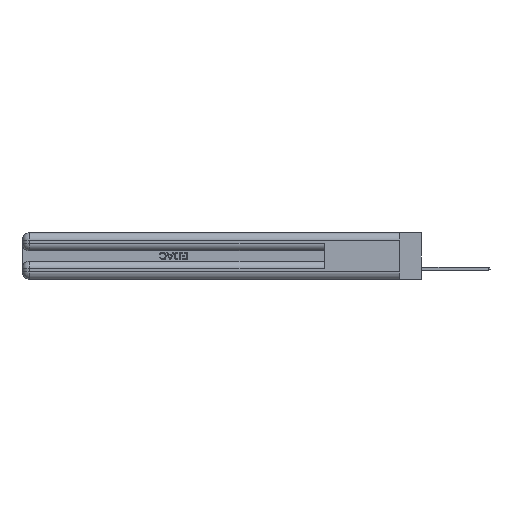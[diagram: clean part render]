
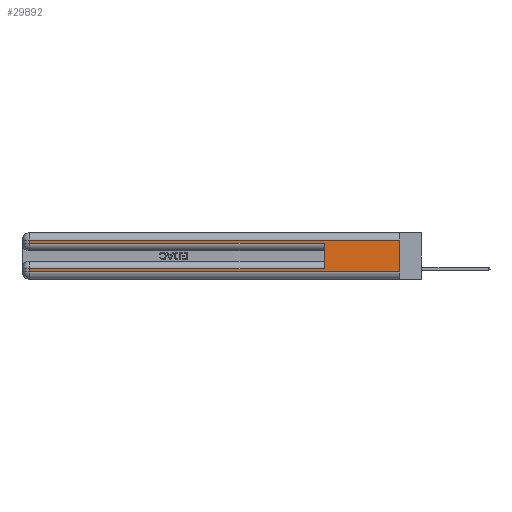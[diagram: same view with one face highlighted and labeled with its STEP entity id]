
A CAD part, left-side view. The second image highlights one B-rep face of the part: STEP entity #29892.
In plain terms, the highlighted planar face has unit normal (-1, 0, 0).
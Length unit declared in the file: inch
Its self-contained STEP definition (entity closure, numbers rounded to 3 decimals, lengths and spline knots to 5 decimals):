
#264 = ORIENTED_EDGE ( 'NONE', *, *, #24487, .T. ) ;
#541 = VECTOR ( 'NONE', #41531, 39.37008 ) ;
#1673 = VERTEX_POINT ( 'NONE', #21031 ) ;
#1889 = ORIENTED_EDGE ( 'NONE', *, *, #11209, .T. ) ;
#2585 = DIRECTION ( 'NONE',  ( 0., 0., 1. ) ) ;
#3064 = EDGE_LOOP ( 'NONE', ( #24831, #13351, #9783, #264, #3946, #1889, #47477, #36276 ) ) ;
#3357 = VECTOR ( 'NONE', #35802, 39.37008 ) ;
#3946 = ORIENTED_EDGE ( 'NONE', *, *, #23975, .F. ) ;
#4025 = DIRECTION ( 'NONE',  ( 1., 0., 0. ) ) ;
#5647 = VERTEX_POINT ( 'NONE', #16318 ) ;
#7057 = DIRECTION ( 'NONE',  ( 0., 0., -1. ) ) ;
#7302 = CARTESIAN_POINT ( 'NONE',  ( 0., 0., 0.37 ) ) ;
#8102 = LINE ( 'NONE', #17677, #43182 ) ;
#8541 = DIRECTION ( 'NONE',  ( 0., 1., 0. ) ) ;
#9783 = ORIENTED_EDGE ( 'NONE', *, *, #28902, .T. ) ;
#10170 = LINE ( 'NONE', #44314, #18719 ) ;
#10703 = CARTESIAN_POINT ( 'NONE',  ( 0., 0., 0.37 ) ) ;
#11209 = EDGE_CURVE ( 'NONE', #25942, #42959, #17731, .T. ) ;
#11585 = CARTESIAN_POINT ( 'NONE',  ( 0., 0., 0.085 ) ) ;
#11626 = LINE ( 'NONE', #10703, #35840 ) ;
#12387 = LINE ( 'NONE', #16403, #26132 ) ;
#13351 = ORIENTED_EDGE ( 'NONE', *, *, #46670, .T. ) ;
#14742 = LINE ( 'NONE', #44589, #44494 ) ;
#16318 = CARTESIAN_POINT ( 'NONE',  ( 0., 0.6, 0.285 ) ) ;
#16403 = CARTESIAN_POINT ( 'NONE',  ( 0., 0., 0.31 ) ) ;
#17677 = CARTESIAN_POINT ( 'NONE',  ( 0., 2.94, 0.37 ) ) ;
#17731 = LINE ( 'NONE', #11585, #3357 ) ;
#18719 = VECTOR ( 'NONE', #7057, 39.37008 ) ;
#20723 = LINE ( 'NONE', #24596, #25910 ) ;
#21031 = CARTESIAN_POINT ( 'NONE',  ( 0., 2.94, 0.285 ) ) ;
#23141 = CARTESIAN_POINT ( 'NONE',  ( 0., 0., 0.31 ) ) ;
#23147 = EDGE_CURVE ( 'NONE', #23586, #42782, #11626, .T. ) ;
#23586 = VERTEX_POINT ( 'NONE', #23141 ) ;
#23975 = EDGE_CURVE ( 'NONE', #25942, #5647, #20723, .T. ) ;
#24487 = EDGE_CURVE ( 'NONE', #1673, #5647, #33379, .T. ) ;
#24596 = CARTESIAN_POINT ( 'NONE',  ( 0., 0.6, 0.145 ) ) ;
#24831 = ORIENTED_EDGE ( 'NONE', *, *, #23147, .F. ) ;
#25293 = VERTEX_POINT ( 'NONE', #38710 ) ;
#25910 = VECTOR ( 'NONE', #2585, 39.37008 ) ;
#25942 = VERTEX_POINT ( 'NONE', #30964 ) ;
#26132 = VECTOR ( 'NONE', #8541, 39.37008 ) ;
#26202 = DIRECTION ( 'NONE',  ( 0., 0., -1. ) ) ;
#28902 = EDGE_CURVE ( 'NONE', #25293, #1673, #8102, .T. ) ;
#29591 = PLANE ( 'NONE',  #45000 ) ;
#29892 = ADVANCED_FACE ( 'NONE', ( #41262 ), #29591, .F. ) ;
#30199 = DIRECTION ( 'NONE',  ( 0., -1., 0. ) ) ;
#30964 = CARTESIAN_POINT ( 'NONE',  ( 0., 0.6, 0.085 ) ) ;
#31677 = EDGE_CURVE ( 'NONE', #42014, #42782, #14742, .T. ) ;
#33269 = CARTESIAN_POINT ( 'NONE',  ( 0., 0., 0.06 ) ) ;
#33291 = DIRECTION ( 'NONE',  ( 0., 0., -1. ) ) ;
#33379 = LINE ( 'NONE', #37541, #541 ) ;
#35577 = CARTESIAN_POINT ( 'NONE',  ( 0., 2.94, 0.06 ) ) ;
#35802 = DIRECTION ( 'NONE',  ( 0., 1., 0. ) ) ;
#35840 = VECTOR ( 'NONE', #26202, 39.37008 ) ;
#36276 = ORIENTED_EDGE ( 'NONE', *, *, #31677, .T. ) ;
#37541 = CARTESIAN_POINT ( 'NONE',  ( 0., 0., 0.285 ) ) ;
#38710 = CARTESIAN_POINT ( 'NONE',  ( 0., 2.94, 0.31 ) ) ;
#41262 = FACE_OUTER_BOUND ( 'NONE', #3064, .T. ) ;
#41362 = CARTESIAN_POINT ( 'NONE',  ( 0., 2.94, 0.085 ) ) ;
#41531 = DIRECTION ( 'NONE',  ( 0., -1., 0. ) ) ;
#42014 = VERTEX_POINT ( 'NONE', #35577 ) ;
#42782 = VERTEX_POINT ( 'NONE', #33269 ) ;
#42959 = VERTEX_POINT ( 'NONE', #41362 ) ;
#43182 = VECTOR ( 'NONE', #46149, 39.37008 ) ;
#44314 = CARTESIAN_POINT ( 'NONE',  ( 0., 2.94, 0.37 ) ) ;
#44494 = VECTOR ( 'NONE', #30199, 39.37008 ) ;
#44589 = CARTESIAN_POINT ( 'NONE',  ( 0., 0., 0.06 ) ) ;
#45000 = AXIS2_PLACEMENT_3D ( 'NONE', #7302, #4025, #33291 ) ;
#46149 = DIRECTION ( 'NONE',  ( 0., 0., -1. ) ) ;
#46347 = EDGE_CURVE ( 'NONE', #42959, #42014, #10170, .T. ) ;
#46670 = EDGE_CURVE ( 'NONE', #23586, #25293, #12387, .T. ) ;
#47477 = ORIENTED_EDGE ( 'NONE', *, *, #46347, .T. ) ;
